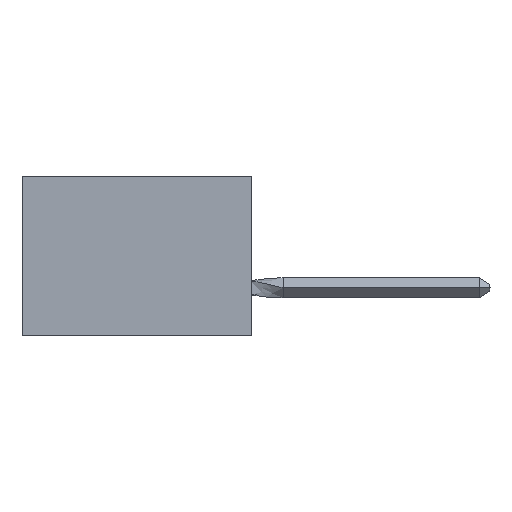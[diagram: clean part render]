
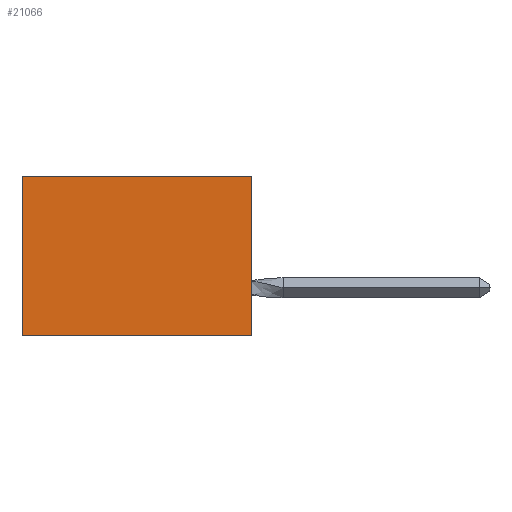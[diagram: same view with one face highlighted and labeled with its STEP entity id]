
A CAD part, left-side view. The second image highlights one B-rep face of the part: STEP entity #21066.
In plain terms, the highlighted planar face has unit normal (-1, 0, 0).
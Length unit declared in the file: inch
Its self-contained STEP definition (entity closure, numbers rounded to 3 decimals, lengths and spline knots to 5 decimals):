
#719 = VERTEX_POINT ( 'NONE', #21634 ) ;
#1254 = EDGE_CURVE ( 'NONE', #32895, #9803, #26858, .T. ) ;
#1932 = DIRECTION ( 'NONE',  ( 1., 0., 0. ) ) ;
#2657 = CARTESIAN_POINT ( 'NONE',  ( 0.305, 0., 0. ) ) ;
#2775 = DIRECTION ( 'NONE',  ( 0., 0., -1. ) ) ;
#2861 = EDGE_CURVE ( 'NONE', #19423, #719, #4041, .T. ) ;
#4041 = LINE ( 'NONE', #33488, #29000 ) ;
#4071 = EDGE_CURVE ( 'NONE', #719, #9803, #7030, .T. ) ;
#6487 = CARTESIAN_POINT ( 'NONE',  ( 0.305, 0.72, -0.5 ) ) ;
#7030 = LINE ( 'NONE', #33403, #30203 ) ;
#7768 = ORIENTED_EDGE ( 'NONE', *, *, #2861, .F. ) ;
#9803 = VERTEX_POINT ( 'NONE', #14235 ) ;
#10290 = ORIENTED_EDGE ( 'NONE', *, *, #4071, .F. ) ;
#10757 = EDGE_LOOP ( 'NONE', ( #14908, #10290, #7768, #11615 ) ) ;
#11615 = ORIENTED_EDGE ( 'NONE', *, *, #24640, .T. ) ;
#12434 = CARTESIAN_POINT ( 'NONE',  ( 0.305, 0.72, 0. ) ) ;
#14235 = CARTESIAN_POINT ( 'NONE',  ( 0.305, 0.72, -0.5 ) ) ;
#14908 = ORIENTED_EDGE ( 'NONE', *, *, #1254, .T. ) ;
#15675 = CARTESIAN_POINT ( 'NONE',  ( 0.305, 0., 0. ) ) ;
#16752 = AXIS2_PLACEMENT_3D ( 'NONE', #27118, #1932, #21375 ) ;
#19042 = DIRECTION ( 'NONE',  ( 0., 1., 0. ) ) ;
#19373 = LINE ( 'NONE', #2657, #29007 ) ;
#19423 = VERTEX_POINT ( 'NONE', #15675 ) ;
#19429 = VECTOR ( 'NONE', #20765, 39.37008 ) ;
#20765 = DIRECTION ( 'NONE',  ( 0., 0., -1. ) ) ;
#21066 = ADVANCED_FACE ( 'NONE', ( #27350 ), #35449, .F. ) ;
#21375 = DIRECTION ( 'NONE',  ( 0., 0., -1. ) ) ;
#21634 = CARTESIAN_POINT ( 'NONE',  ( 0.305, 0., -0.5 ) ) ;
#22376 = DIRECTION ( 'NONE',  ( 0., 1., 0. ) ) ;
#24640 = EDGE_CURVE ( 'NONE', #19423, #32895, #19373, .T. ) ;
#26858 = LINE ( 'NONE', #6487, #19429 ) ;
#27118 = CARTESIAN_POINT ( 'NONE',  ( 0.305, 0., -0.5 ) ) ;
#27350 = FACE_OUTER_BOUND ( 'NONE', #10757, .T. ) ;
#29000 = VECTOR ( 'NONE', #2775, 39.37008 ) ;
#29007 = VECTOR ( 'NONE', #19042, 39.37008 ) ;
#30203 = VECTOR ( 'NONE', #22376, 39.37008 ) ;
#32895 = VERTEX_POINT ( 'NONE', #12434 ) ;
#33403 = CARTESIAN_POINT ( 'NONE',  ( 0.305, 0., -0.5 ) ) ;
#33488 = CARTESIAN_POINT ( 'NONE',  ( 0.305, 0., -0.5 ) ) ;
#35449 = PLANE ( 'NONE',  #16752 ) ;
